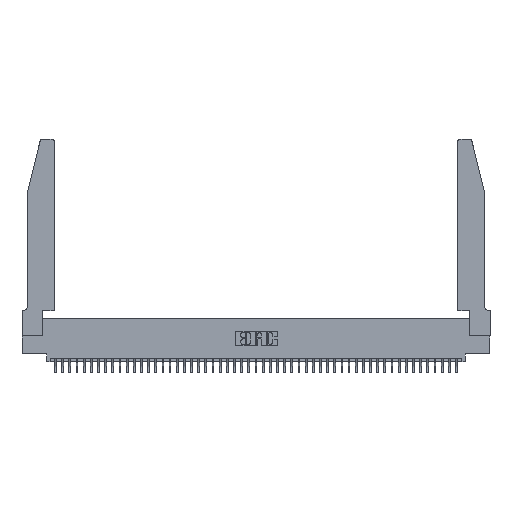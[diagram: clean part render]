
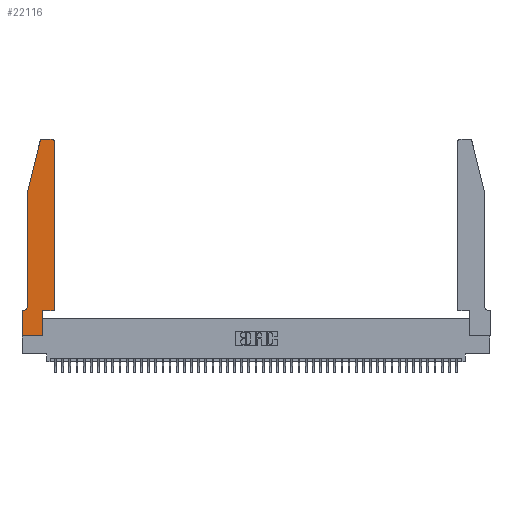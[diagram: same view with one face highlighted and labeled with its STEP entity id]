
A CAD part, top view. The second image highlights one B-rep face of the part: STEP entity #22116.
In plain terms, the highlighted planar face has unit normal (0, 0, 1).
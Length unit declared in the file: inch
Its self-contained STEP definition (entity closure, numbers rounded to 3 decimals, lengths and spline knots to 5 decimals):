
#724 = VERTEX_POINT ( 'NONE', #21389 ) ;
#973 = VERTEX_POINT ( 'NONE', #27685 ) ;
#1806 = CARTESIAN_POINT ( 'NONE',  ( 0.2865, 0., 0.37 ) ) ;
#2618 = VERTEX_POINT ( 'NONE', #6147 ) ;
#2629 = DIRECTION ( 'NONE',  ( 0., 0., 1. ) ) ;
#2930 = CIRCLE ( 'NONE', #14413, 0.07 ) ;
#3084 = CARTESIAN_POINT ( 'NONE',  ( 0.0055, 0.42, 0.37 ) ) ;
#3099 = CARTESIAN_POINT ( 'NONE',  ( 0.284, 2.72, 0.37 ) ) ;
#3183 = VERTEX_POINT ( 'NONE', #27962 ) ;
#3888 = CARTESIAN_POINT ( 'NONE',  ( 0.4505, 0.35, 0.37 ) ) ;
#3922 = LINE ( 'NONE', #45298, #32839 ) ;
#4104 = VERTEX_POINT ( 'NONE', #37043 ) ;
#4296 = CARTESIAN_POINT ( 'NONE',  ( 0., 0., 0.37 ) ) ;
#4301 = EDGE_CURVE ( 'NONE', #6287, #724, #3922, .T. ) ;
#4995 = CARTESIAN_POINT ( 'NONE',  ( 0., 0., 0.37 ) ) ;
#6147 = CARTESIAN_POINT ( 'NONE',  ( 0.25487, 2.72718, 0.37 ) ) ;
#6287 = VERTEX_POINT ( 'NONE', #1806 ) ;
#6573 = ORIENTED_EDGE ( 'NONE', *, *, #6574, .T. ) ;
#6574 = EDGE_CURVE ( 'NONE', #973, #12112, #30312, .T. ) ;
#6593 = CARTESIAN_POINT ( 'NONE',  ( 0.4505, 2.72, 0.37 ) ) ;
#7957 = EDGE_LOOP ( 'NONE', ( #6573, #39850, #33449, #14171, #13153, #39259, #30803, #16136, #39173, #22259, #33128, #42563 ) ) ;
#9143 = EDGE_CURVE ( 'NONE', #25609, #46456, #2930, .T. ) ;
#10227 = EDGE_CURVE ( 'NONE', #36200, #973, #38685, .T. ) ;
#10351 = DIRECTION ( 'NONE',  ( -1., 0., 0. ) ) ;
#10548 = DIRECTION ( 'NONE',  ( 1., 0., 0. ) ) ;
#11965 = DIRECTION ( 'NONE',  ( 0., -1., 0. ) ) ;
#12112 = VERTEX_POINT ( 'NONE', #23514 ) ;
#13153 = ORIENTED_EDGE ( 'NONE', *, *, #9143, .T. ) ;
#13490 = EDGE_CURVE ( 'NONE', #42018, #36200, #26796, .T. ) ;
#14171 = ORIENTED_EDGE ( 'NONE', *, *, #21975, .T. ) ;
#14413 = AXIS2_PLACEMENT_3D ( 'NONE', #3084, #28976, #47207 ) ;
#14688 = LINE ( 'NONE', #47493, #36054 ) ;
#16105 = CARTESIAN_POINT ( 'NONE',  ( 0.4205, 2.72, 0.37 ) ) ;
#16136 = ORIENTED_EDGE ( 'NONE', *, *, #41981, .T. ) ;
#16719 = VECTOR ( 'NONE', #40403, 39.37008 ) ;
#16872 = FACE_OUTER_BOUND ( 'NONE', #7957, .T. ) ;
#16917 = VECTOR ( 'NONE', #37585, 39.37008 ) ;
#17514 = AXIS2_PLACEMENT_3D ( 'NONE', #16105, #30509, #41942 ) ;
#17929 = EDGE_CURVE ( 'NONE', #12112, #2618, #34566, .T. ) ;
#19288 = DIRECTION ( 'NONE',  ( 0., 1., 0. ) ) ;
#20535 = EDGE_CURVE ( 'NONE', #46456, #4104, #14688, .T. ) ;
#21389 = CARTESIAN_POINT ( 'NONE',  ( 0.2865, 0.35, 0.37 ) ) ;
#21975 = EDGE_CURVE ( 'NONE', #3183, #25609, #32557, .T. ) ;
#22046 = VECTOR ( 'NONE', #44395, 39.37008 ) ;
#22116 = ADVANCED_FACE ( 'NONE', ( #16872 ), #32600, .T. ) ;
#22259 = ORIENTED_EDGE ( 'NONE', *, *, #39752, .T. ) ;
#22824 = LINE ( 'NONE', #4995, #44216 ) ;
#22929 = CARTESIAN_POINT ( 'NONE',  ( 0.4505, 0.35, 0.37 ) ) ;
#23085 = DIRECTION ( 'NONE',  ( 0., 1., 0. ) ) ;
#23208 = LINE ( 'NONE', #33105, #22046 ) ;
#23314 = VERTEX_POINT ( 'NONE', #35554 ) ;
#23514 = CARTESIAN_POINT ( 'NONE',  ( 0.284, 2.75, 0.37 ) ) ;
#25200 = AXIS2_PLACEMENT_3D ( 'NONE', #47135, #29213, #36297 ) ;
#25411 = LINE ( 'NONE', #3888, #16719 ) ;
#25609 = VERTEX_POINT ( 'NONE', #43772 ) ;
#26796 = LINE ( 'NONE', #22929, #38896 ) ;
#27685 = CARTESIAN_POINT ( 'NONE',  ( 0.4205, 2.75, 0.37 ) ) ;
#27962 = CARTESIAN_POINT ( 'NONE',  ( 0.0755, 2., 0.37 ) ) ;
#28117 = EDGE_CURVE ( 'NONE', #4104, #23314, #22824, .T. ) ;
#28976 = DIRECTION ( 'NONE',  ( 0., 0., -1. ) ) ;
#29213 = DIRECTION ( 'NONE',  ( 0., 0., 1. ) ) ;
#29925 = CARTESIAN_POINT ( 'NONE',  ( 0.2605, 2.75, 0.37 ) ) ;
#30090 = DIRECTION ( 'NONE',  ( -1., 0., 0. ) ) ;
#30201 = CARTESIAN_POINT ( 'NONE',  ( 0.0755, 2., 0.37 ) ) ;
#30312 = LINE ( 'NONE', #29925, #38943 ) ;
#30509 = DIRECTION ( 'NONE',  ( 0., 0., 1. ) ) ;
#30803 = ORIENTED_EDGE ( 'NONE', *, *, #28117, .T. ) ;
#31968 = AXIS2_PLACEMENT_3D ( 'NONE', #3099, #2629, #10548 ) ;
#32557 = LINE ( 'NONE', #30201, #16917 ) ;
#32600 = PLANE ( 'NONE',  #25200 ) ;
#32839 = VECTOR ( 'NONE', #19288, 39.37008 ) ;
#33105 = CARTESIAN_POINT ( 'NONE',  ( 0.0755, 2., 0.37 ) ) ;
#33128 = ORIENTED_EDGE ( 'NONE', *, *, #13490, .T. ) ;
#33449 = ORIENTED_EDGE ( 'NONE', *, *, #38152, .T. ) ;
#34566 = CIRCLE ( 'NONE', #31968, 0.03 ) ;
#35554 = CARTESIAN_POINT ( 'NONE',  ( 0., 0., 0.37 ) ) ;
#36054 = VECTOR ( 'NONE', #10351, 39.37008 ) ;
#36200 = VERTEX_POINT ( 'NONE', #6593 ) ;
#36297 = DIRECTION ( 'NONE',  ( 1., 0., 0. ) ) ;
#37043 = CARTESIAN_POINT ( 'NONE',  ( 0., 0.35, 0.37 ) ) ;
#37077 = CARTESIAN_POINT ( 'NONE',  ( 0.4505, 0.35, 0.37 ) ) ;
#37585 = DIRECTION ( 'NONE',  ( 0., -1., 0. ) ) ;
#38152 = EDGE_CURVE ( 'NONE', #2618, #3183, #23208, .T. ) ;
#38685 = CIRCLE ( 'NONE', #17514, 0.03 ) ;
#38896 = VECTOR ( 'NONE', #23085, 39.37008 ) ;
#38943 = VECTOR ( 'NONE', #30090, 39.37008 ) ;
#39002 = LINE ( 'NONE', #4296, #43039 ) ;
#39173 = ORIENTED_EDGE ( 'NONE', *, *, #4301, .T. ) ;
#39259 = ORIENTED_EDGE ( 'NONE', *, *, #20535, .T. ) ;
#39752 = EDGE_CURVE ( 'NONE', #724, #42018, #25411, .T. ) ;
#39850 = ORIENTED_EDGE ( 'NONE', *, *, #17929, .T. ) ;
#40403 = DIRECTION ( 'NONE',  ( 1., 0., 0. ) ) ;
#41942 = DIRECTION ( 'NONE',  ( 1., 0., 0. ) ) ;
#41981 = EDGE_CURVE ( 'NONE', #23314, #6287, #39002, .T. ) ;
#42018 = VERTEX_POINT ( 'NONE', #37077 ) ;
#42563 = ORIENTED_EDGE ( 'NONE', *, *, #10227, .T. ) ;
#43039 = VECTOR ( 'NONE', #44695, 39.37008 ) ;
#43256 = CARTESIAN_POINT ( 'NONE',  ( 0.0055, 0.35, 0.37 ) ) ;
#43772 = CARTESIAN_POINT ( 'NONE',  ( 0.0755, 0.42, 0.37 ) ) ;
#44216 = VECTOR ( 'NONE', #11965, 39.37008 ) ;
#44395 = DIRECTION ( 'NONE',  ( -0.239, -0.971, 0. ) ) ;
#44695 = DIRECTION ( 'NONE',  ( 1., 0., 0. ) ) ;
#45298 = CARTESIAN_POINT ( 'NONE',  ( 0.2865, 0.35, 0.37 ) ) ;
#46456 = VERTEX_POINT ( 'NONE', #43256 ) ;
#47135 = CARTESIAN_POINT ( 'NONE',  ( 0., 0.35, 0.37 ) ) ;
#47207 = DIRECTION ( 'NONE',  ( -1., 0., 0. ) ) ;
#47493 = CARTESIAN_POINT ( 'NONE',  ( 0.0755, 0.35, 0.37 ) ) ;
